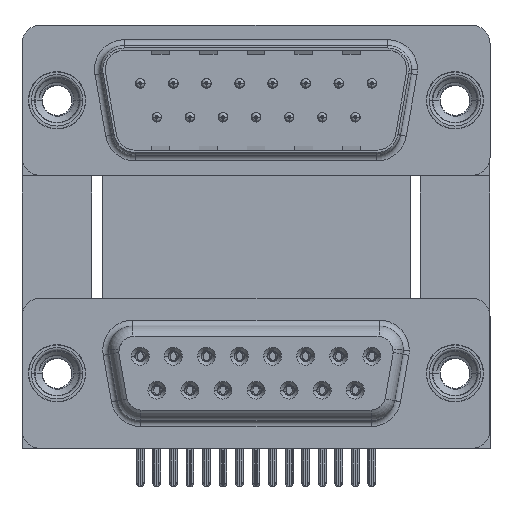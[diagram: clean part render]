
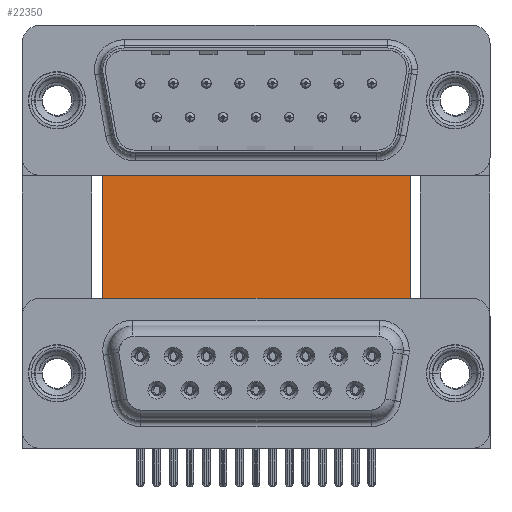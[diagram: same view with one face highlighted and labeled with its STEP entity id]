
A CAD part, top view. The second image highlights one B-rep face of the part: STEP entity #22350.
In plain terms, the highlighted planar face has unit normal (0, 0, 1).
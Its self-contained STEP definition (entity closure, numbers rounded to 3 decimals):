
#1004 = CARTESIAN_POINT ( 'NONE',  ( 3.79, 16.585, -12. ) ) ;
#2736 = VERTEX_POINT ( 'NONE', #32982 ) ;
#2962 = VECTOR ( 'NONE', #45663, 1000. ) ;
#3354 = LINE ( 'NONE', #32524, #39643 ) ;
#5340 = VERTEX_POINT ( 'NONE', #41900 ) ;
#6914 = CARTESIAN_POINT ( 'NONE',  ( 3.79, -3.735, -12. ) ) ;
#7081 = LINE ( 'NONE', #42849, #2962 ) ;
#7549 = CARTESIAN_POINT ( 'NONE',  ( 3.79, 16.585, -12. ) ) ;
#8925 = ORIENTED_EDGE ( 'NONE', *, *, #44778, .T. ) ;
#9133 = CARTESIAN_POINT ( 'NONE',  ( 29.58, 16.585, -12. ) ) ;
#11840 = LINE ( 'NONE', #1004, #14247 ) ;
#13605 = VERTEX_POINT ( 'NONE', #9133 ) ;
#14139 = DIRECTION ( 'NONE',  ( 0., 0., -1. ) ) ;
#14175 = VERTEX_POINT ( 'NONE', #6914 ) ;
#14247 = VECTOR ( 'NONE', #36299, 1000. ) ;
#16988 = EDGE_CURVE ( 'NONE', #2736, #13605, #11840, .T. ) ;
#17236 = EDGE_CURVE ( 'NONE', #2736, #14175, #7081, .T. ) ;
#22350 = ADVANCED_FACE ( 'NONE', ( #38839 ), #25154, .F. ) ;
#25154 = PLANE ( 'NONE',  #42442 ) ;
#25936 = VECTOR ( 'NONE', #41369, 1000. ) ;
#27439 = LINE ( 'NONE', #38513, #25936 ) ;
#28929 = DIRECTION ( 'NONE',  ( -1., 0., 0. ) ) ;
#32524 = CARTESIAN_POINT ( 'NONE',  ( 3.79, -3.735, -12. ) ) ;
#32982 = CARTESIAN_POINT ( 'NONE',  ( 3.79, 16.585, -12. ) ) ;
#33856 = ORIENTED_EDGE ( 'NONE', *, *, #40871, .F. ) ;
#34969 = ORIENTED_EDGE ( 'NONE', *, *, #16988, .F. ) ;
#36299 = DIRECTION ( 'NONE',  ( 1., 0., 0. ) ) ;
#37179 = EDGE_LOOP ( 'NONE', ( #8925, #33856, #34969, #41796 ) ) ;
#38513 = CARTESIAN_POINT ( 'NONE',  ( 29.58, 16.585, -12. ) ) ;
#38839 = FACE_OUTER_BOUND ( 'NONE', #37179, .T. ) ;
#39643 = VECTOR ( 'NONE', #39807, 1000. ) ;
#39807 = DIRECTION ( 'NONE',  ( 1., 0., 0. ) ) ;
#40871 = EDGE_CURVE ( 'NONE', #13605, #5340, #27439, .T. ) ;
#41369 = DIRECTION ( 'NONE',  ( 0., -1., 0. ) ) ;
#41796 = ORIENTED_EDGE ( 'NONE', *, *, #17236, .T. ) ;
#41900 = CARTESIAN_POINT ( 'NONE',  ( 29.58, -3.735, -12. ) ) ;
#42442 = AXIS2_PLACEMENT_3D ( 'NONE', #7549, #14139, #28929 ) ;
#42849 = CARTESIAN_POINT ( 'NONE',  ( 3.79, 16.585, -12. ) ) ;
#44778 = EDGE_CURVE ( 'NONE', #14175, #5340, #3354, .T. ) ;
#45663 = DIRECTION ( 'NONE',  ( 0., -1., 0. ) ) ;
